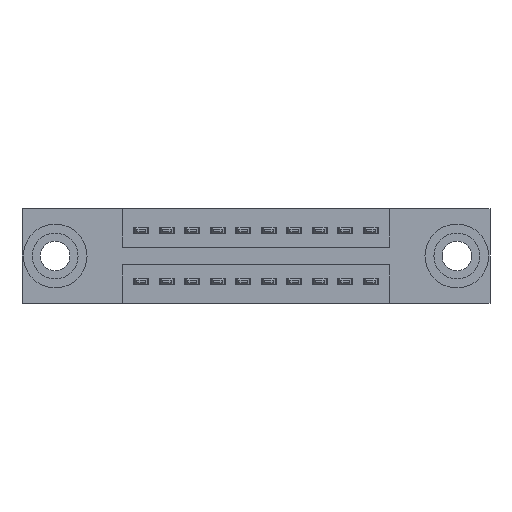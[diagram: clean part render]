
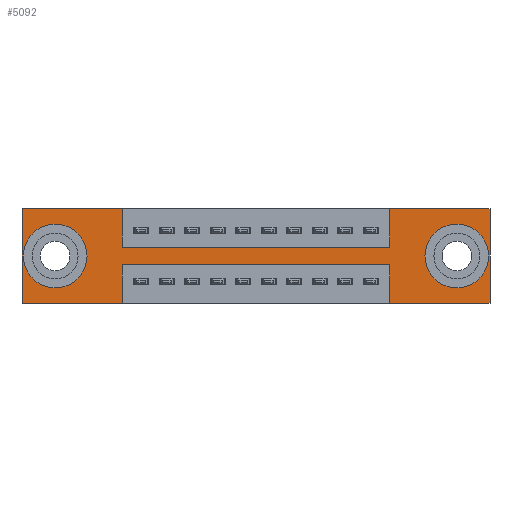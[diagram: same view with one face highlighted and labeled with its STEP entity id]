
A CAD part, front view. The second image highlights one B-rep face of the part: STEP entity #5092.
In plain terms, the highlighted planar face has unit normal (0, -1, 0).
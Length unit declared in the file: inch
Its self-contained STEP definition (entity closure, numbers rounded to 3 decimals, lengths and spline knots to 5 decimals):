
#79 = AXIS2_PLACEMENT_3D ( 'NONE', #8209, #11974, #296 ) ;
#121 = DIRECTION ( 'NONE',  ( 0., 0., 1. ) ) ;
#231 = ORIENTED_EDGE ( 'NONE', *, *, #3156, .F. ) ;
#285 = DIRECTION ( 'NONE',  ( 0., 0., -1. ) ) ;
#296 = DIRECTION ( 'NONE',  ( 0., 0., 1. ) ) ;
#318 = ORIENTED_EDGE ( 'NONE', *, *, #977, .T. ) ;
#501 = CIRCLE ( 'NONE', #79, 0.078 ) ;
#564 = LINE ( 'NONE', #6115, #8501 ) ;
#613 = ORIENTED_EDGE ( 'NONE', *, *, #7465, .F. ) ;
#622 = LINE ( 'NONE', #2024, #3394 ) ;
#746 = EDGE_LOOP ( 'NONE', ( #3895, #2013 ) ) ;
#764 = CARTESIAN_POINT ( 'NONE',  ( 1.835, 0., -0.37 ) ) ;
#800 = EDGE_CURVE ( 'NONE', #3422, #4125, #5318, .T. ) ;
#853 = CIRCLE ( 'NONE', #7906, 0.078 ) ;
#946 = ORIENTED_EDGE ( 'NONE', *, *, #7848, .F. ) ;
#973 = EDGE_CURVE ( 'NONE', #11434, #3422, #564, .T. ) ;
#977 = EDGE_CURVE ( 'NONE', #2931, #1709, #853, .T. ) ;
#1117 = VERTEX_POINT ( 'NONE', #11342 ) ;
#1260 = CARTESIAN_POINT ( 'NONE',  ( 0.13, 0., -0.185 ) ) ;
#1324 = CARTESIAN_POINT ( 'NONE',  ( 1.835, 0., 0. ) ) ;
#1511 = EDGE_LOOP ( 'NONE', ( #318, #7755 ) ) ;
#1597 = ORIENTED_EDGE ( 'NONE', *, *, #8413, .F. ) ;
#1709 = VERTEX_POINT ( 'NONE', #4027 ) ;
#1815 = VERTEX_POINT ( 'NONE', #1987 ) ;
#1841 = EDGE_CURVE ( 'NONE', #6006, #1117, #6809, .T. ) ;
#1848 = EDGE_CURVE ( 'NONE', #9437, #7202, #10333, .T. ) ;
#1851 = EDGE_CURVE ( 'NONE', #2247, #6159, #12306, .T. ) ;
#1918 = EDGE_CURVE ( 'NONE', #6489, #1815, #6504, .T. ) ;
#1987 = CARTESIAN_POINT ( 'NONE',  ( 0.13, 0., -0.107 ) ) ;
#2013 = ORIENTED_EDGE ( 'NONE', *, *, #1918, .T. ) ;
#2024 = CARTESIAN_POINT ( 'NONE',  ( 0.3925, 0., -0.15 ) ) ;
#2247 = VERTEX_POINT ( 'NONE', #4081 ) ;
#2285 = VECTOR ( 'NONE', #4461, 39.37008 ) ;
#2370 = DIRECTION ( 'NONE',  ( 0., 0., 1. ) ) ;
#2393 = CARTESIAN_POINT ( 'NONE',  ( 1.705, 0., -0.185 ) ) ;
#2432 = ORIENTED_EDGE ( 'NONE', *, *, #1851, .F. ) ;
#2644 = ORIENTED_EDGE ( 'NONE', *, *, #973, .F. ) ;
#2670 = ORIENTED_EDGE ( 'NONE', *, *, #10531, .F. ) ;
#2827 = ORIENTED_EDGE ( 'NONE', *, *, #11065, .F. ) ;
#2923 = CARTESIAN_POINT ( 'NONE',  ( 0.3925, 0., 0. ) ) ;
#2931 = VERTEX_POINT ( 'NONE', #7917 ) ;
#3095 = DIRECTION ( 'NONE',  ( -1., 0., 0. ) ) ;
#3156 = EDGE_CURVE ( 'NONE', #9396, #7759, #5861, .T. ) ;
#3234 = FACE_BOUND ( 'NONE', #746, .T. ) ;
#3257 = CARTESIAN_POINT ( 'NONE',  ( 1.4425, 0., -0.22 ) ) ;
#3394 = VECTOR ( 'NONE', #6811, 39.37008 ) ;
#3422 = VERTEX_POINT ( 'NONE', #5084 ) ;
#3502 = CARTESIAN_POINT ( 'NONE',  ( 0., 0., -0.37 ) ) ;
#3699 = CARTESIAN_POINT ( 'NONE',  ( 0.3925, 0., -0.15 ) ) ;
#3751 = VECTOR ( 'NONE', #10445, 39.37008 ) ;
#3871 = CARTESIAN_POINT ( 'NONE',  ( 0., 0., 0. ) ) ;
#3895 = ORIENTED_EDGE ( 'NONE', *, *, #6962, .T. ) ;
#4027 = CARTESIAN_POINT ( 'NONE',  ( 1.705, 0., -0.263 ) ) ;
#4081 = CARTESIAN_POINT ( 'NONE',  ( 0.3925, 0., 0. ) ) ;
#4117 = DIRECTION ( 'NONE',  ( 0., 1., 0. ) ) ;
#4125 = VERTEX_POINT ( 'NONE', #1324 ) ;
#4199 = CARTESIAN_POINT ( 'NONE',  ( 0.13, 0., -0.263 ) ) ;
#4358 = CARTESIAN_POINT ( 'NONE',  ( 0., 0., 0. ) ) ;
#4461 = DIRECTION ( 'NONE',  ( -1., 0., 0. ) ) ;
#4862 = LINE ( 'NONE', #3502, #2285 ) ;
#5084 = CARTESIAN_POINT ( 'NONE',  ( 1.4425, 0., 0. ) ) ;
#5092 = ADVANCED_FACE ( 'NONE', ( #7783, #3234, #7649 ), #10288, .T. ) ;
#5106 = VECTOR ( 'NONE', #2370, 39.37008 ) ;
#5176 = CARTESIAN_POINT ( 'NONE',  ( 0., 0., 0. ) ) ;
#5262 = LINE ( 'NONE', #7258, #5106 ) ;
#5318 = LINE ( 'NONE', #5176, #11561 ) ;
#5861 = LINE ( 'NONE', #10534, #3751 ) ;
#5985 = DIRECTION ( 'NONE',  ( 0., 0., -1. ) ) ;
#6006 = VERTEX_POINT ( 'NONE', #7545 ) ;
#6036 = VECTOR ( 'NONE', #5985, 39.37008 ) ;
#6104 = DIRECTION ( 'NONE',  ( 1., 0., 0. ) ) ;
#6107 = LINE ( 'NONE', #7950, #9181 ) ;
#6115 = CARTESIAN_POINT ( 'NONE',  ( 1.4425, 0., 0. ) ) ;
#6159 = VERTEX_POINT ( 'NONE', #3699 ) ;
#6200 = DIRECTION ( 'NONE',  ( 0., 0., -1. ) ) ;
#6277 = DIRECTION ( 'NONE',  ( 0., 1., 0. ) ) ;
#6378 = AXIS2_PLACEMENT_3D ( 'NONE', #1260, #8079, #9086 ) ;
#6381 = CARTESIAN_POINT ( 'NONE',  ( 0., 0., 0. ) ) ;
#6489 = VERTEX_POINT ( 'NONE', #4199 ) ;
#6504 = CIRCLE ( 'NONE', #6378, 0.078 ) ;
#6724 = VECTOR ( 'NONE', #11030, 39.37008 ) ;
#6809 = LINE ( 'NONE', #8828, #6036 ) ;
#6811 = DIRECTION ( 'NONE',  ( 1., 0., 0. ) ) ;
#6817 = DIRECTION ( 'NONE',  ( 0., 0., -1. ) ) ;
#6962 = EDGE_CURVE ( 'NONE', #1815, #6489, #501, .T. ) ;
#7018 = AXIS2_PLACEMENT_3D ( 'NONE', #10369, #8305, #7388 ) ;
#7169 = DIRECTION ( 'NONE',  ( 0., 0., -1. ) ) ;
#7202 = VERTEX_POINT ( 'NONE', #6381 ) ;
#7258 = CARTESIAN_POINT ( 'NONE',  ( 1.4425, 0., -0.37 ) ) ;
#7388 = DIRECTION ( 'NONE',  ( 0., 0., -1. ) ) ;
#7462 = CIRCLE ( 'NONE', #9833, 0.078 ) ;
#7465 = EDGE_CURVE ( 'NONE', #6159, #11434, #622, .T. ) ;
#7545 = CARTESIAN_POINT ( 'NONE',  ( 0.3925, 0., -0.22 ) ) ;
#7649 = FACE_OUTER_BOUND ( 'NONE', #9698, .T. ) ;
#7675 = VERTEX_POINT ( 'NONE', #3257 ) ;
#7747 = ORIENTED_EDGE ( 'NONE', *, *, #1841, .F. ) ;
#7755 = ORIENTED_EDGE ( 'NONE', *, *, #9588, .T. ) ;
#7759 = VERTEX_POINT ( 'NONE', #10561 ) ;
#7783 = FACE_BOUND ( 'NONE', #1511, .T. ) ;
#7848 = EDGE_CURVE ( 'NONE', #7202, #2247, #11763, .T. ) ;
#7857 = VECTOR ( 'NONE', #3095, 39.37008 ) ;
#7906 = AXIS2_PLACEMENT_3D ( 'NONE', #8984, #4117, #285 ) ;
#7917 = CARTESIAN_POINT ( 'NONE',  ( 1.705, 0., -0.107 ) ) ;
#7950 = CARTESIAN_POINT ( 'NONE',  ( 1.835, 0., 0. ) ) ;
#8079 = DIRECTION ( 'NONE',  ( 0., 1., 0. ) ) ;
#8122 = DIRECTION ( 'NONE',  ( 0., 0., 1. ) ) ;
#8209 = CARTESIAN_POINT ( 'NONE',  ( 0.13, 0., -0.185 ) ) ;
#8305 = DIRECTION ( 'NONE',  ( 0., -1., 0. ) ) ;
#8351 = CARTESIAN_POINT ( 'NONE',  ( 0.3925, 0., -0.22 ) ) ;
#8413 = EDGE_CURVE ( 'NONE', #4125, #9396, #6107, .T. ) ;
#8432 = EDGE_CURVE ( 'NONE', #1117, #9437, #4862, .T. ) ;
#8501 = VECTOR ( 'NONE', #8122, 39.37008 ) ;
#8708 = CARTESIAN_POINT ( 'NONE',  ( 1.4425, 0., -0.15 ) ) ;
#8828 = CARTESIAN_POINT ( 'NONE',  ( 0.3925, 0., -0.37 ) ) ;
#8885 = ORIENTED_EDGE ( 'NONE', *, *, #800, .F. ) ;
#8984 = CARTESIAN_POINT ( 'NONE',  ( 1.705, 0., -0.185 ) ) ;
#9012 = CARTESIAN_POINT ( 'NONE',  ( 0., 0., -0.37 ) ) ;
#9086 = DIRECTION ( 'NONE',  ( 0., 0., 1. ) ) ;
#9181 = VECTOR ( 'NONE', #7169, 39.37008 ) ;
#9396 = VERTEX_POINT ( 'NONE', #764 ) ;
#9437 = VERTEX_POINT ( 'NONE', #9012 ) ;
#9512 = ORIENTED_EDGE ( 'NONE', *, *, #8432, .F. ) ;
#9588 = EDGE_CURVE ( 'NONE', #1709, #2931, #7462, .T. ) ;
#9698 = EDGE_LOOP ( 'NONE', ( #7747, #2670, #2827, #231, #1597, #8885, #2644, #613, #2432, #946, #10639, #9512 ) ) ;
#9718 = VECTOR ( 'NONE', #6817, 39.37008 ) ;
#9833 = AXIS2_PLACEMENT_3D ( 'NONE', #2393, #6277, #6200 ) ;
#9866 = LINE ( 'NONE', #8351, #7857 ) ;
#10288 = PLANE ( 'NONE',  #7018 ) ;
#10333 = LINE ( 'NONE', #3871, #11538 ) ;
#10369 = CARTESIAN_POINT ( 'NONE',  ( 0., 0., -0.37 ) ) ;
#10445 = DIRECTION ( 'NONE',  ( -1., 0., 0. ) ) ;
#10531 = EDGE_CURVE ( 'NONE', #7675, #6006, #9866, .T. ) ;
#10534 = CARTESIAN_POINT ( 'NONE',  ( 0., 0., -0.37 ) ) ;
#10561 = CARTESIAN_POINT ( 'NONE',  ( 1.4425, 0., -0.37 ) ) ;
#10639 = ORIENTED_EDGE ( 'NONE', *, *, #1848, .F. ) ;
#11030 = DIRECTION ( 'NONE',  ( 1., 0., 0. ) ) ;
#11065 = EDGE_CURVE ( 'NONE', #7759, #7675, #5262, .T. ) ;
#11342 = CARTESIAN_POINT ( 'NONE',  ( 0.3925, 0., -0.37 ) ) ;
#11434 = VERTEX_POINT ( 'NONE', #8708 ) ;
#11538 = VECTOR ( 'NONE', #121, 39.37008 ) ;
#11561 = VECTOR ( 'NONE', #6104, 39.37008 ) ;
#11763 = LINE ( 'NONE', #4358, #6724 ) ;
#11974 = DIRECTION ( 'NONE',  ( 0., 1., 0. ) ) ;
#12306 = LINE ( 'NONE', #2923, #9718 ) ;
